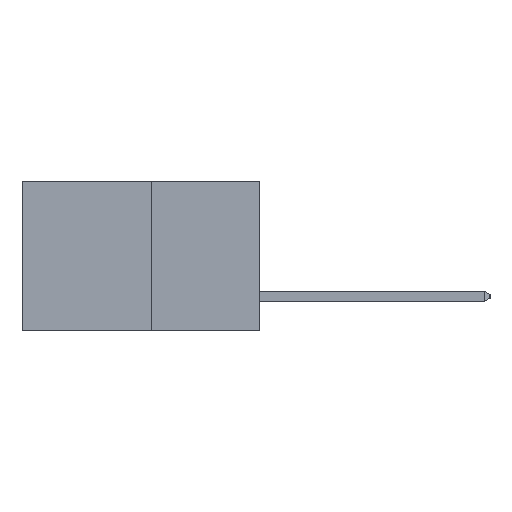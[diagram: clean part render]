
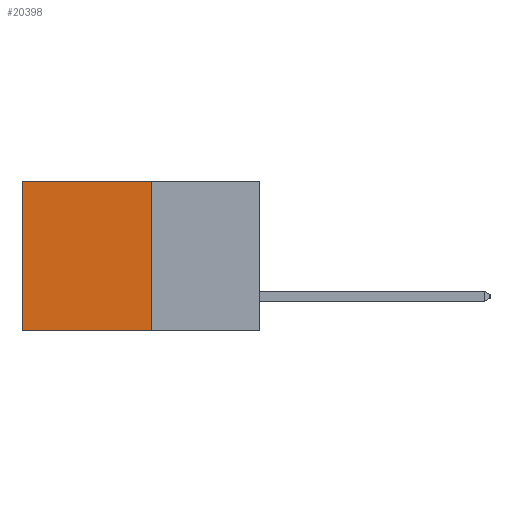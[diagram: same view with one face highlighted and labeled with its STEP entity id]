
A CAD part, left-side view. The second image highlights one B-rep face of the part: STEP entity #20398.
In plain terms, the highlighted planar face has unit normal (-1, 0, 0).
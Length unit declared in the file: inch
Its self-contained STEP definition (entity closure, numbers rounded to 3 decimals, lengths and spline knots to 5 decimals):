
#928 = VERTEX_POINT ( 'NONE', #7583 ) ;
#2565 = CARTESIAN_POINT ( 'NONE',  ( 0.277, 0.59, -0.37 ) ) ;
#3956 = DIRECTION ( 'NONE',  ( 0., 0., -1. ) ) ;
#4225 = VECTOR ( 'NONE', #3956, 39.37008 ) ;
#4447 = CARTESIAN_POINT ( 'NONE',  ( 0.277, 0.27, 0. ) ) ;
#4474 = DIRECTION ( 'NONE',  ( 0., 0., -1. ) ) ;
#4802 = CARTESIAN_POINT ( 'NONE',  ( 0.277, 0.27, -0.37 ) ) ;
#5672 = CARTESIAN_POINT ( 'NONE',  ( 0.277, 0.59, -0.37 ) ) ;
#6010 = ORIENTED_EDGE ( 'NONE', *, *, #18163, .T. ) ;
#6521 = EDGE_CURVE ( 'NONE', #21824, #928, #6893, .T. ) ;
#6583 = DIRECTION ( 'NONE',  ( 0., 1., 0. ) ) ;
#6883 = VECTOR ( 'NONE', #6583, 39.37008 ) ;
#6893 = LINE ( 'NONE', #18430, #20687 ) ;
#7583 = CARTESIAN_POINT ( 'NONE',  ( 0.277, 0.59, 0. ) ) ;
#7598 = ORIENTED_EDGE ( 'NONE', *, *, #12148, .F. ) ;
#8222 = AXIS2_PLACEMENT_3D ( 'NONE', #9481, #9566, #21975 ) ;
#8639 = LINE ( 'NONE', #2565, #23316 ) ;
#8677 = FACE_OUTER_BOUND ( 'NONE', #8986, .T. ) ;
#8986 = EDGE_LOOP ( 'NONE', ( #6010, #10000, #7598, #16161 ) ) ;
#9182 = CARTESIAN_POINT ( 'NONE',  ( 0.277, 0.27, -0.37 ) ) ;
#9481 = CARTESIAN_POINT ( 'NONE',  ( 0.277, 0.27, -0.37 ) ) ;
#9566 = DIRECTION ( 'NONE',  ( 1., 0., 0. ) ) ;
#10000 = ORIENTED_EDGE ( 'NONE', *, *, #21277, .F. ) ;
#12148 = EDGE_CURVE ( 'NONE', #21824, #14001, #14724, .T. ) ;
#14001 = VERTEX_POINT ( 'NONE', #9182 ) ;
#14724 = LINE ( 'NONE', #20222, #4225 ) ;
#15013 = DIRECTION ( 'NONE',  ( 0., 1., 0. ) ) ;
#16161 = ORIENTED_EDGE ( 'NONE', *, *, #6521, .T. ) ;
#16988 = VERTEX_POINT ( 'NONE', #5672 ) ;
#18163 = EDGE_CURVE ( 'NONE', #928, #16988, #8639, .T. ) ;
#18430 = CARTESIAN_POINT ( 'NONE',  ( 0.277, 0.27, 0. ) ) ;
#18567 = PLANE ( 'NONE',  #8222 ) ;
#20222 = CARTESIAN_POINT ( 'NONE',  ( 0.277, 0.27, -0.37 ) ) ;
#20398 = ADVANCED_FACE ( 'NONE', ( #8677 ), #18567, .F. ) ;
#20679 = LINE ( 'NONE', #4802, #6883 ) ;
#20687 = VECTOR ( 'NONE', #15013, 39.37008 ) ;
#21277 = EDGE_CURVE ( 'NONE', #14001, #16988, #20679, .T. ) ;
#21824 = VERTEX_POINT ( 'NONE', #4447 ) ;
#21975 = DIRECTION ( 'NONE',  ( 0., 0., -1. ) ) ;
#23316 = VECTOR ( 'NONE', #4474, 39.37008 ) ;
